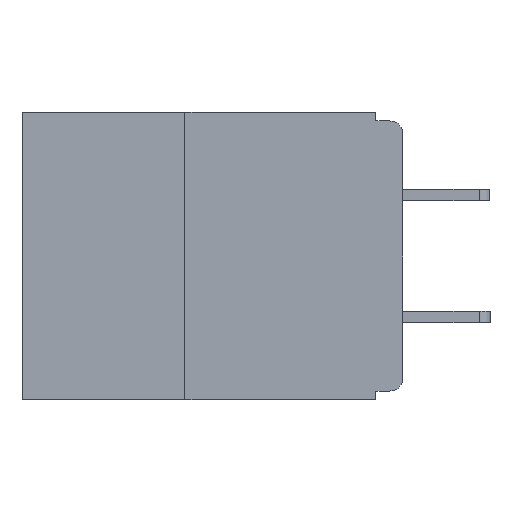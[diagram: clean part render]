
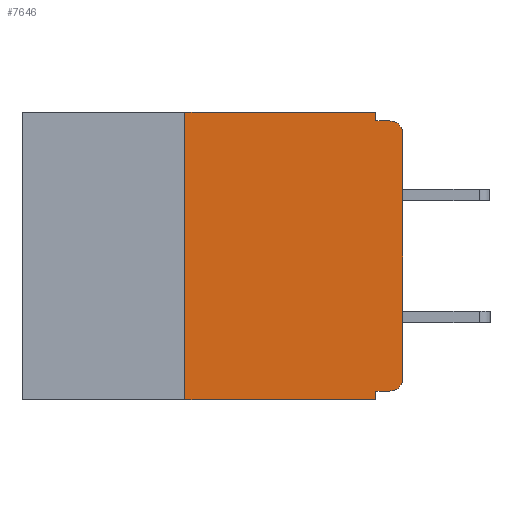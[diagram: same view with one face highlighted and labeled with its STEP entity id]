
A CAD part, left-side view. The second image highlights one B-rep face of the part: STEP entity #7646.
In plain terms, the highlighted planar face has unit normal (-1, 0, 0).
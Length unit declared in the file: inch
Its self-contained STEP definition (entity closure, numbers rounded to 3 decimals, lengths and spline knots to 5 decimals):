
#339 = VERTEX_POINT ( 'NONE', #9248 ) ;
#655 = CARTESIAN_POINT ( 'NONE',  ( 0., 0.25, -0.33 ) ) ;
#679 = VECTOR ( 'NONE', #8622, 39.37008 ) ;
#1039 = DIRECTION ( 'NONE',  ( 0., -1., 0. ) ) ;
#1638 = VECTOR ( 'NONE', #5733, 39.37008 ) ;
#1708 = CARTESIAN_POINT ( 'NONE',  ( 0., 0.015, -0.025 ) ) ;
#1812 = EDGE_CURVE ( 'NONE', #9569, #21417, #9896, .T. ) ;
#2024 = CARTESIAN_POINT ( 'NONE',  ( 0., 0.031, -0.33 ) ) ;
#2342 = LINE ( 'NONE', #5654, #20537 ) ;
#2567 = CARTESIAN_POINT ( 'NONE',  ( 0., 0., -0.305 ) ) ;
#2891 = LINE ( 'NONE', #18735, #7218 ) ;
#3083 = CARTESIAN_POINT ( 'NONE',  ( 0., 0.031, -0.01 ) ) ;
#3549 = VERTEX_POINT ( 'NONE', #14097 ) ;
#3701 = VECTOR ( 'NONE', #15074, 39.37008 ) ;
#4136 = CARTESIAN_POINT ( 'NONE',  ( 0., 0.015, -0.32 ) ) ;
#4222 = VERTEX_POINT ( 'NONE', #22681 ) ;
#4266 = ORIENTED_EDGE ( 'NONE', *, *, #15644, .F. ) ;
#4367 = CARTESIAN_POINT ( 'NONE',  ( 0., 0.031, 0. ) ) ;
#5323 = DIRECTION ( 'NONE',  ( 0., 1., 0. ) ) ;
#5421 = ORIENTED_EDGE ( 'NONE', *, *, #6754, .F. ) ;
#5654 = CARTESIAN_POINT ( 'NONE',  ( 0., 0., -0.32 ) ) ;
#5733 = DIRECTION ( 'NONE',  ( 0., 0., 1. ) ) ;
#5740 = DIRECTION ( 'NONE',  ( -1., 0., 0. ) ) ;
#5821 = LINE ( 'NONE', #19299, #10638 ) ;
#5892 = CARTESIAN_POINT ( 'NONE',  ( 0., 0.437, 0. ) ) ;
#6150 = LINE ( 'NONE', #20638, #679 ) ;
#6534 = LINE ( 'NONE', #7513, #1638 ) ;
#6754 = EDGE_CURVE ( 'NONE', #18306, #339, #2342, .T. ) ;
#6875 = ORIENTED_EDGE ( 'NONE', *, *, #21854, .T. ) ;
#7218 = VECTOR ( 'NONE', #1039, 39.37008 ) ;
#7448 = ORIENTED_EDGE ( 'NONE', *, *, #1812, .T. ) ;
#7513 = CARTESIAN_POINT ( 'NONE',  ( 0., 0., 0. ) ) ;
#7646 = ADVANCED_FACE ( 'NONE', ( #8321 ), #16936, .F. ) ;
#8012 = ORIENTED_EDGE ( 'NONE', *, *, #16791, .F. ) ;
#8321 = FACE_OUTER_BOUND ( 'NONE', #20438, .T. ) ;
#8568 = ORIENTED_EDGE ( 'NONE', *, *, #10506, .F. ) ;
#8590 = LINE ( 'NONE', #655, #3701 ) ;
#8622 = DIRECTION ( 'NONE',  ( 0., 0., -1. ) ) ;
#9248 = CARTESIAN_POINT ( 'NONE',  ( 0., 0.031, -0.32 ) ) ;
#9569 = VERTEX_POINT ( 'NONE', #22265 ) ;
#9896 = CIRCLE ( 'NONE', #15366, 0.015 ) ;
#10207 = VECTOR ( 'NONE', #16901, 39.37008 ) ;
#10506 = EDGE_CURVE ( 'NONE', #3549, #18367, #11312, .T. ) ;
#10638 = VECTOR ( 'NONE', #10727, 39.37008 ) ;
#10727 = DIRECTION ( 'NONE',  ( 0., -1., 0. ) ) ;
#11285 = DIRECTION ( 'NONE',  ( 0., -1., 0. ) ) ;
#11312 = LINE ( 'NONE', #5892, #15409 ) ;
#12157 = EDGE_CURVE ( 'NONE', #339, #22395, #6150, .T. ) ;
#12776 = EDGE_CURVE ( 'NONE', #16975, #21417, #5821, .T. ) ;
#13317 = AXIS2_PLACEMENT_3D ( 'NONE', #16371, #5740, #18063 ) ;
#13850 = ORIENTED_EDGE ( 'NONE', *, *, #14458, .T. ) ;
#14097 = CARTESIAN_POINT ( 'NONE',  ( 0., 0.25, 0. ) ) ;
#14369 = ORIENTED_EDGE ( 'NONE', *, *, #12157, .F. ) ;
#14458 = EDGE_CURVE ( 'NONE', #4222, #22395, #2891, .T. ) ;
#14871 = LINE ( 'NONE', #15178, #10207 ) ;
#14918 = ORIENTED_EDGE ( 'NONE', *, *, #20022, .T. ) ;
#15074 = DIRECTION ( 'NONE',  ( 0., 0., 1. ) ) ;
#15115 = CARTESIAN_POINT ( 'NONE',  ( 0., 0.015, -0.01 ) ) ;
#15178 = CARTESIAN_POINT ( 'NONE',  ( 0., 0.031, 0. ) ) ;
#15366 = AXIS2_PLACEMENT_3D ( 'NONE', #1708, #20913, #18062 ) ;
#15409 = VECTOR ( 'NONE', #11285, 39.37008 ) ;
#15413 = AXIS2_PLACEMENT_3D ( 'NONE', #17675, #16915, #16888 ) ;
#15644 = EDGE_CURVE ( 'NONE', #4222, #3549, #8590, .T. ) ;
#16371 = CARTESIAN_POINT ( 'NONE',  ( 0., 0.015, -0.305 ) ) ;
#16791 = EDGE_CURVE ( 'NONE', #18367, #16975, #14871, .T. ) ;
#16888 = DIRECTION ( 'NONE',  ( 0., 0., -1. ) ) ;
#16901 = DIRECTION ( 'NONE',  ( 0., 0., -1. ) ) ;
#16915 = DIRECTION ( 'NONE',  ( 1., 0., 0. ) ) ;
#16936 = PLANE ( 'NONE',  #15413 ) ;
#16975 = VERTEX_POINT ( 'NONE', #3083 ) ;
#17424 = CIRCLE ( 'NONE', #13317, 0.015 ) ;
#17675 = CARTESIAN_POINT ( 'NONE',  ( 0., 0.437, 0. ) ) ;
#18062 = DIRECTION ( 'NONE',  ( 0., 0., -1. ) ) ;
#18063 = DIRECTION ( 'NONE',  ( 0., 0., -1. ) ) ;
#18306 = VERTEX_POINT ( 'NONE', #4136 ) ;
#18367 = VERTEX_POINT ( 'NONE', #4367 ) ;
#18735 = CARTESIAN_POINT ( 'NONE',  ( 0., 0.437, -0.33 ) ) ;
#19299 = CARTESIAN_POINT ( 'NONE',  ( 0., 0., -0.01 ) ) ;
#19513 = VERTEX_POINT ( 'NONE', #2567 ) ;
#20022 = EDGE_CURVE ( 'NONE', #18306, #19513, #17424, .T. ) ;
#20438 = EDGE_LOOP ( 'NONE', ( #6875, #7448, #21261, #8012, #8568, #4266, #13850, #14369, #5421, #14918 ) ) ;
#20537 = VECTOR ( 'NONE', #5323, 39.37008 ) ;
#20638 = CARTESIAN_POINT ( 'NONE',  ( 0., 0.031, -0.33 ) ) ;
#20913 = DIRECTION ( 'NONE',  ( -1., 0., 0. ) ) ;
#21261 = ORIENTED_EDGE ( 'NONE', *, *, #12776, .F. ) ;
#21417 = VERTEX_POINT ( 'NONE', #15115 ) ;
#21854 = EDGE_CURVE ( 'NONE', #19513, #9569, #6534, .T. ) ;
#22265 = CARTESIAN_POINT ( 'NONE',  ( 0., 0., -0.025 ) ) ;
#22395 = VERTEX_POINT ( 'NONE', #2024 ) ;
#22681 = CARTESIAN_POINT ( 'NONE',  ( 0., 0.25, -0.33 ) ) ;
